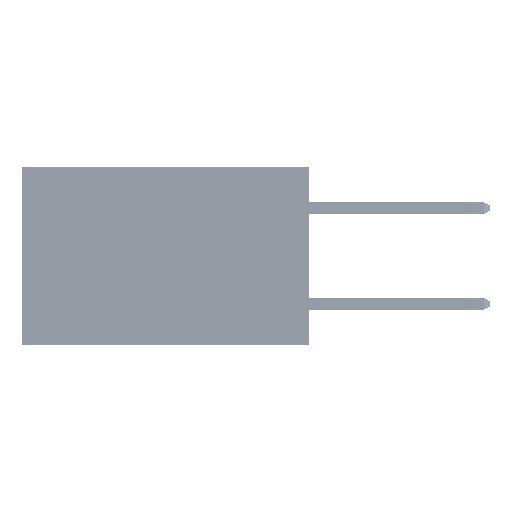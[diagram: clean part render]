
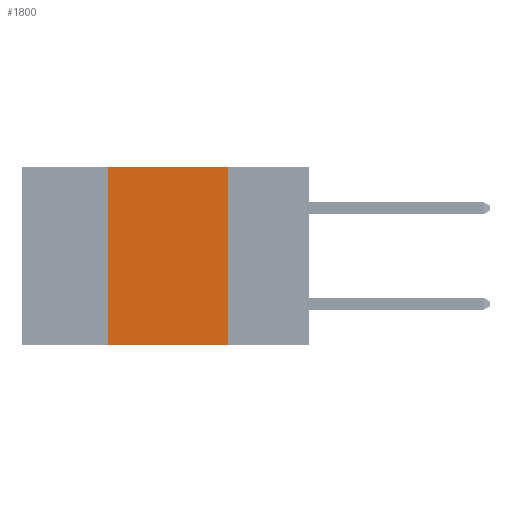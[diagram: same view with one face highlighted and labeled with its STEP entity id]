
A CAD part, left-side view. The second image highlights one B-rep face of the part: STEP entity #1800.
In plain terms, the highlighted planar face has unit normal (-1, 0, 0).
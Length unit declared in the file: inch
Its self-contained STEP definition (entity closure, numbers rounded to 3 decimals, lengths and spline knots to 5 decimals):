
#1276 = CARTESIAN_POINT ( 'NONE',  ( 0., 0.42, -0.37 ) ) ;
#1800 = ADVANCED_FACE ( 'NONE', ( #24411 ), #31425, .F. ) ;
#1866 = AXIS2_PLACEMENT_3D ( 'NONE', #20047, #40225, #48094 ) ;
#3487 = ORIENTED_EDGE ( 'NONE', *, *, #24993, .F. ) ;
#4557 = CARTESIAN_POINT ( 'NONE',  ( 0., 0.17, 0. ) ) ;
#7105 = ORIENTED_EDGE ( 'NONE', *, *, #38342, .T. ) ;
#7471 = VERTEX_POINT ( 'NONE', #15099 ) ;
#7968 = DIRECTION ( 'NONE',  ( 0., -1., 0. ) ) ;
#8371 = VECTOR ( 'NONE', #7968, 39.37008 ) ;
#14919 = CARTESIAN_POINT ( 'NONE',  ( 0., 0.6, 0. ) ) ;
#15099 = CARTESIAN_POINT ( 'NONE',  ( 0., 0.17, 0. ) ) ;
#16050 = CARTESIAN_POINT ( 'NONE',  ( 0., 0.6, -0.37 ) ) ;
#16494 = EDGE_LOOP ( 'NONE', ( #48314, #3487, #19703, #7105 ) ) ;
#17514 = LINE ( 'NONE', #33944, #50128 ) ;
#19016 = LINE ( 'NONE', #4557, #20250 ) ;
#19703 = ORIENTED_EDGE ( 'NONE', *, *, #46154, .F. ) ;
#20047 = CARTESIAN_POINT ( 'NONE',  ( 0., 0.6, 0. ) ) ;
#20250 = VECTOR ( 'NONE', #21094, 39.37008 ) ;
#21094 = DIRECTION ( 'NONE',  ( 0., 0., -1. ) ) ;
#24411 = FACE_OUTER_BOUND ( 'NONE', #16494, .T. ) ;
#24993 = EDGE_CURVE ( 'NONE', #49314, #7471, #36345, .T. ) ;
#26218 = CARTESIAN_POINT ( 'NONE',  ( 0., 0.17, -0.37 ) ) ;
#26350 = VECTOR ( 'NONE', #34724, 39.37008 ) ;
#28096 = EDGE_CURVE ( 'NONE', #7471, #44786, #19016, .T. ) ;
#31425 = PLANE ( 'NONE',  #1866 ) ;
#33704 = VERTEX_POINT ( 'NONE', #1276 ) ;
#33944 = CARTESIAN_POINT ( 'NONE',  ( 0., 0.42, 0. ) ) ;
#34724 = DIRECTION ( 'NONE',  ( 0., -1., 0. ) ) ;
#35990 = LINE ( 'NONE', #16050, #8371 ) ;
#36345 = LINE ( 'NONE', #14919, #26350 ) ;
#38342 = EDGE_CURVE ( 'NONE', #33704, #44786, #35990, .T. ) ;
#40171 = CARTESIAN_POINT ( 'NONE',  ( 0., 0.42, 0. ) ) ;
#40225 = DIRECTION ( 'NONE',  ( 1., 0., 0. ) ) ;
#42070 = DIRECTION ( 'NONE',  ( 0., 0., 1. ) ) ;
#44786 = VERTEX_POINT ( 'NONE', #26218 ) ;
#46154 = EDGE_CURVE ( 'NONE', #33704, #49314, #17514, .T. ) ;
#48094 = DIRECTION ( 'NONE',  ( 0., 0., -1. ) ) ;
#48314 = ORIENTED_EDGE ( 'NONE', *, *, #28096, .F. ) ;
#49314 = VERTEX_POINT ( 'NONE', #40171 ) ;
#50128 = VECTOR ( 'NONE', #42070, 39.37008 ) ;
